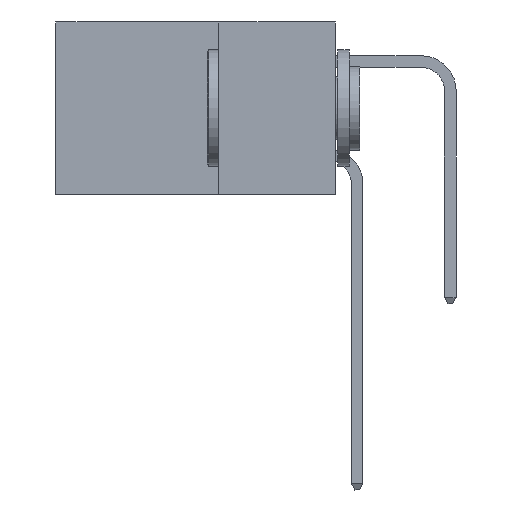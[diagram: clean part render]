
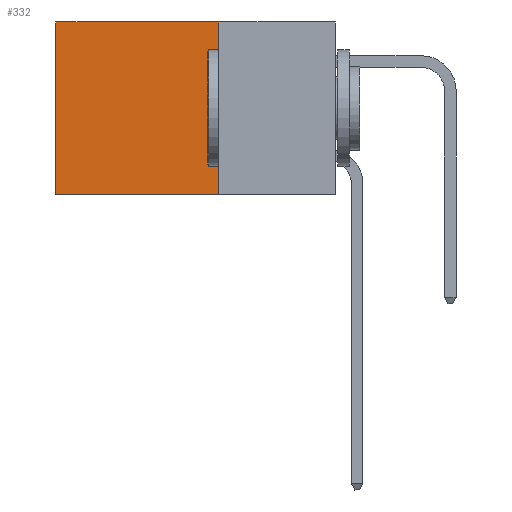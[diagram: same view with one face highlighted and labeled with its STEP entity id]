
A CAD part, left-side view. The second image highlights one B-rep face of the part: STEP entity #332.
In plain terms, the highlighted planar face has unit normal (-1, 0, 0).
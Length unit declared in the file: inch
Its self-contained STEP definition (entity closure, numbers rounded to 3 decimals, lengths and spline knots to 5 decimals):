
#332 = ADVANCED_FACE ( 'NONE', ( #35851 ), #17863, .F. ) ;
#3356 = EDGE_LOOP ( 'NONE', ( #4992, #40920, #15411, #9287 ) ) ;
#3432 = CARTESIAN_POINT ( 'NONE',  ( 0.2875, 0.6, 0. ) ) ;
#3494 = CARTESIAN_POINT ( 'NONE',  ( 0.2875, 0.25, 0. ) ) ;
#4992 = ORIENTED_EDGE ( 'NONE', *, *, #8862, .T. ) ;
#7831 = DIRECTION ( 'NONE',  ( 1., 0., 0. ) ) ;
#8110 = DIRECTION ( 'NONE',  ( 0., 0., -1. ) ) ;
#8862 = EDGE_CURVE ( 'NONE', #30823, #28065, #20313, .T. ) ;
#9287 = ORIENTED_EDGE ( 'NONE', *, *, #30988, .T. ) ;
#13730 = CARTESIAN_POINT ( 'NONE',  ( 0.2875, 0.25, 0. ) ) ;
#15411 = ORIENTED_EDGE ( 'NONE', *, *, #17401, .F. ) ;
#17401 = EDGE_CURVE ( 'NONE', #34259, #31611, #37341, .T. ) ;
#17644 = VECTOR ( 'NONE', #31021, 39.37008 ) ;
#17863 = PLANE ( 'NONE',  #25589 ) ;
#18172 = CARTESIAN_POINT ( 'NONE',  ( 0.2875, 0.25, 0. ) ) ;
#20313 = LINE ( 'NONE', #3432, #31068 ) ;
#21200 = CARTESIAN_POINT ( 'NONE',  ( 0.2875, 0.6, 0. ) ) ;
#21309 = CARTESIAN_POINT ( 'NONE',  ( 0.2875, 0.25, -0.37 ) ) ;
#23261 = LINE ( 'NONE', #21309, #17644 ) ;
#25411 = EDGE_CURVE ( 'NONE', #31611, #28065, #23261, .T. ) ;
#25589 = AXIS2_PLACEMENT_3D ( 'NONE', #27745, #7831, #8110 ) ;
#27614 = VECTOR ( 'NONE', #39331, 39.37008 ) ;
#27745 = CARTESIAN_POINT ( 'NONE',  ( 0.2875, 0.25, 0. ) ) ;
#27961 = VECTOR ( 'NONE', #41481, 39.37008 ) ;
#28065 = VERTEX_POINT ( 'NONE', #41644 ) ;
#30823 = VERTEX_POINT ( 'NONE', #21200 ) ;
#30988 = EDGE_CURVE ( 'NONE', #34259, #30823, #37672, .T. ) ;
#31021 = DIRECTION ( 'NONE',  ( 0., 1., 0. ) ) ;
#31068 = VECTOR ( 'NONE', #32824, 39.37008 ) ;
#31611 = VERTEX_POINT ( 'NONE', #38388 ) ;
#32824 = DIRECTION ( 'NONE',  ( 0., 0., -1. ) ) ;
#34259 = VERTEX_POINT ( 'NONE', #13730 ) ;
#35851 = FACE_OUTER_BOUND ( 'NONE', #3356, .T. ) ;
#37341 = LINE ( 'NONE', #3494, #27614 ) ;
#37672 = LINE ( 'NONE', #18172, #27961 ) ;
#38388 = CARTESIAN_POINT ( 'NONE',  ( 0.2875, 0.25, -0.37 ) ) ;
#39331 = DIRECTION ( 'NONE',  ( 0., 0., -1. ) ) ;
#40920 = ORIENTED_EDGE ( 'NONE', *, *, #25411, .F. ) ;
#41481 = DIRECTION ( 'NONE',  ( 0., 1., 0. ) ) ;
#41644 = CARTESIAN_POINT ( 'NONE',  ( 0.2875, 0.6, -0.37 ) ) ;
